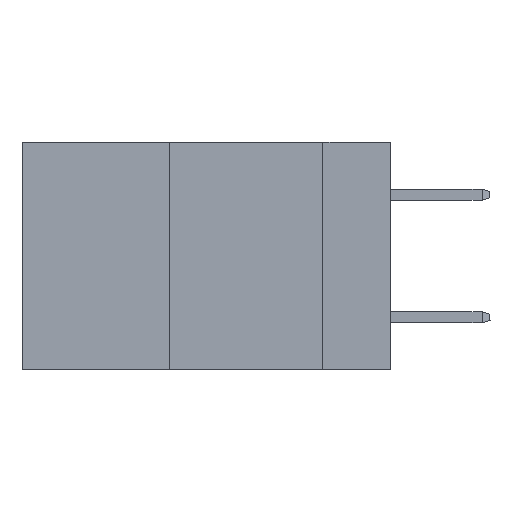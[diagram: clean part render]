
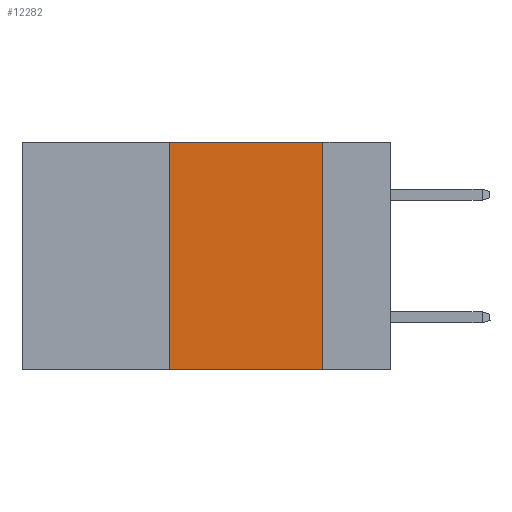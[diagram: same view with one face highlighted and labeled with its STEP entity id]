
A CAD part, left-side view. The second image highlights one B-rep face of the part: STEP entity #12282.
In plain terms, the highlighted planar face has unit normal (-1, 0, 0).
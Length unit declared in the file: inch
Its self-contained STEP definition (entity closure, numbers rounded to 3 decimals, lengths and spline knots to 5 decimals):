
#254 = LINE ( 'NONE', #22393, #18183 ) ;
#2164 = CARTESIAN_POINT ( 'NONE',  ( 0., 0.11, 0. ) ) ;
#2251 = EDGE_CURVE ( 'NONE', #5272, #11071, #6532, .T. ) ;
#2308 = CARTESIAN_POINT ( 'NONE',  ( 0., 0.36, -0.37 ) ) ;
#2878 = CARTESIAN_POINT ( 'NONE',  ( 0., 0.6, 0. ) ) ;
#2955 = CARTESIAN_POINT ( 'NONE',  ( 0., 0.6, 0. ) ) ;
#4082 = DIRECTION ( 'NONE',  ( 0., 0., -1. ) ) ;
#4154 = EDGE_CURVE ( 'NONE', #11071, #14751, #23583, .T. ) ;
#4454 = ORIENTED_EDGE ( 'NONE', *, *, #21660, .F. ) ;
#4690 = ORIENTED_EDGE ( 'NONE', *, *, #4154, .F. ) ;
#4800 = ORIENTED_EDGE ( 'NONE', *, *, #2251, .F. ) ;
#4844 = DIRECTION ( 'NONE',  ( 0., 0., -1. ) ) ;
#4914 = ORIENTED_EDGE ( 'NONE', *, *, #14676, .T. ) ;
#5272 = VERTEX_POINT ( 'NONE', #2308 ) ;
#5591 = AXIS2_PLACEMENT_3D ( 'NONE', #2955, #15838, #4844 ) ;
#6056 = DIRECTION ( 'NONE',  ( 0., -1., 0. ) ) ;
#6532 = LINE ( 'NONE', #13223, #10283 ) ;
#6680 = VERTEX_POINT ( 'NONE', #13183 ) ;
#7812 = DIRECTION ( 'NONE',  ( 0., 0., 1. ) ) ;
#7875 = EDGE_LOOP ( 'NONE', ( #4454, #4690, #4800, #4914 ) ) ;
#8577 = DIRECTION ( 'NONE',  ( 0., -1., 0. ) ) ;
#10283 = VECTOR ( 'NONE', #7812, 39.37008 ) ;
#10387 = PLANE ( 'NONE',  #5591 ) ;
#11071 = VERTEX_POINT ( 'NONE', #16909 ) ;
#12282 = ADVANCED_FACE ( 'NONE', ( #15426 ), #10387, .F. ) ;
#13183 = CARTESIAN_POINT ( 'NONE',  ( 0., 0.11, -0.37 ) ) ;
#13223 = CARTESIAN_POINT ( 'NONE',  ( 0., 0.36, 0. ) ) ;
#13514 = CARTESIAN_POINT ( 'NONE',  ( 0., 0.11, 0. ) ) ;
#14676 = EDGE_CURVE ( 'NONE', #5272, #6680, #254, .T. ) ;
#14751 = VERTEX_POINT ( 'NONE', #13514 ) ;
#15426 = FACE_OUTER_BOUND ( 'NONE', #7875, .T. ) ;
#15838 = DIRECTION ( 'NONE',  ( 1., 0., 0. ) ) ;
#16909 = CARTESIAN_POINT ( 'NONE',  ( 0., 0.36, 0. ) ) ;
#16972 = VECTOR ( 'NONE', #4082, 39.37008 ) ;
#17572 = LINE ( 'NONE', #2164, #16972 ) ;
#18183 = VECTOR ( 'NONE', #6056, 39.37008 ) ;
#18737 = VECTOR ( 'NONE', #8577, 39.37008 ) ;
#21660 = EDGE_CURVE ( 'NONE', #14751, #6680, #17572, .T. ) ;
#22393 = CARTESIAN_POINT ( 'NONE',  ( 0., 0.6, -0.37 ) ) ;
#23583 = LINE ( 'NONE', #2878, #18737 ) ;
